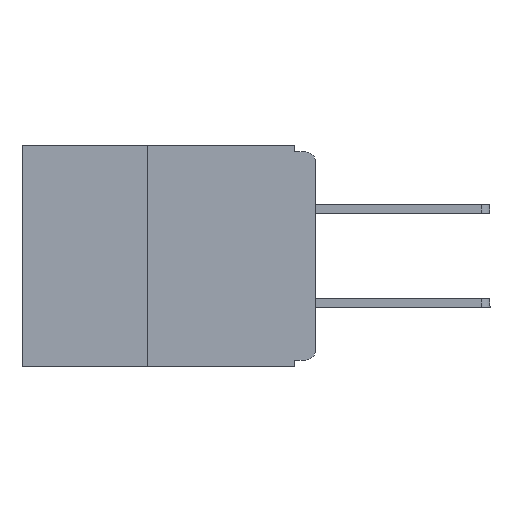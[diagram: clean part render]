
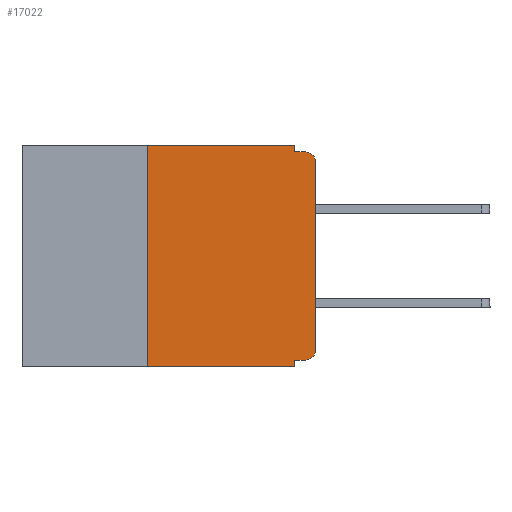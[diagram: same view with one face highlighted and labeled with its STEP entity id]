
A CAD part, left-side view. The second image highlights one B-rep face of the part: STEP entity #17022.
In plain terms, the highlighted planar face has unit normal (-1, 0, 0).
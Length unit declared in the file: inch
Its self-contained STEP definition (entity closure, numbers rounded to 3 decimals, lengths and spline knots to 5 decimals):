
#171 = DIRECTION ( 'NONE',  ( 0., 0., 1. ) ) ;
#229 = VERTEX_POINT ( 'NONE', #3097 ) ;
#685 = CARTESIAN_POINT ( 'NONE',  ( 0., 0., -0.305 ) ) ;
#747 = VERTEX_POINT ( 'NONE', #20195 ) ;
#1390 = ORIENTED_EDGE ( 'NONE', *, *, #5855, .T. ) ;
#1569 = PLANE ( 'NONE',  #25095 ) ;
#1769 = EDGE_CURVE ( 'NONE', #11417, #20608, #27484, .T. ) ;
#2028 = LINE ( 'NONE', #30187, #28240 ) ;
#2188 = EDGE_CURVE ( 'NONE', #27932, #9509, #2028, .T. ) ;
#2592 = LINE ( 'NONE', #24137, #16158 ) ;
#2807 = CIRCLE ( 'NONE', #29738, 0.015 ) ;
#3097 = CARTESIAN_POINT ( 'NONE',  ( 0., 0.031, -0.33 ) ) ;
#3810 = EDGE_CURVE ( 'NONE', #20608, #4296, #27402, .T. ) ;
#4108 = DIRECTION ( 'NONE',  ( 1., 0., 0. ) ) ;
#4151 = LINE ( 'NONE', #15385, #30288 ) ;
#4296 = VERTEX_POINT ( 'NONE', #9428 ) ;
#5158 = ORIENTED_EDGE ( 'NONE', *, *, #30270, .F. ) ;
#5855 = EDGE_CURVE ( 'NONE', #11417, #229, #32579, .T. ) ;
#6663 = CARTESIAN_POINT ( 'NONE',  ( 0., 0.25, -0.33 ) ) ;
#7225 = DIRECTION ( 'NONE',  ( -1., 0., 0. ) ) ;
#8771 = ORIENTED_EDGE ( 'NONE', *, *, #2188, .F. ) ;
#9335 = VERTEX_POINT ( 'NONE', #32453 ) ;
#9428 = CARTESIAN_POINT ( 'NONE',  ( 0., 0.031, 0. ) ) ;
#9509 = VERTEX_POINT ( 'NONE', #30810 ) ;
#9636 = ORIENTED_EDGE ( 'NONE', *, *, #11539, .T. ) ;
#10554 = FACE_OUTER_BOUND ( 'NONE', #23819, .T. ) ;
#10931 = DIRECTION ( 'NONE',  ( -1., 0., 0. ) ) ;
#11417 = VERTEX_POINT ( 'NONE', #6663 ) ;
#11539 = EDGE_CURVE ( 'NONE', #27932, #21836, #19241, .T. ) ;
#11646 = CARTESIAN_POINT ( 'NONE',  ( 0., 0.437, 0. ) ) ;
#12445 = CARTESIAN_POINT ( 'NONE',  ( 0., 0., -0.01 ) ) ;
#12714 = VECTOR ( 'NONE', #19038, 39.37008 ) ;
#12812 = CARTESIAN_POINT ( 'NONE',  ( 0., 0.031, -0.01 ) ) ;
#13519 = LINE ( 'NONE', #26538, #12714 ) ;
#13847 = VECTOR ( 'NONE', #20989, 39.37008 ) ;
#14106 = DIRECTION ( 'NONE',  ( 0., 1., 0. ) ) ;
#14584 = EDGE_CURVE ( 'NONE', #15882, #9335, #21091, .T. ) ;
#15385 = CARTESIAN_POINT ( 'NONE',  ( 0., 0., 0. ) ) ;
#15882 = VERTEX_POINT ( 'NONE', #12812 ) ;
#16158 = VECTOR ( 'NONE', #26626, 39.37008 ) ;
#16305 = ORIENTED_EDGE ( 'NONE', *, *, #14584, .F. ) ;
#17022 = ADVANCED_FACE ( 'NONE', ( #10554 ), #1569, .F. ) ;
#17591 = CARTESIAN_POINT ( 'NONE',  ( 0., 0.015, -0.32 ) ) ;
#19038 = DIRECTION ( 'NONE',  ( 0., 0., -1. ) ) ;
#19241 = CIRCLE ( 'NONE', #24144, 0.015 ) ;
#20195 = CARTESIAN_POINT ( 'NONE',  ( 0., 0., -0.025 ) ) ;
#20608 = VERTEX_POINT ( 'NONE', #26088 ) ;
#20829 = VECTOR ( 'NONE', #23068, 39.37008 ) ;
#20943 = CARTESIAN_POINT ( 'NONE',  ( 0., 0.437, 0. ) ) ;
#20989 = DIRECTION ( 'NONE',  ( 0., -1., 0. ) ) ;
#21091 = LINE ( 'NONE', #12445, #23723 ) ;
#21836 = VERTEX_POINT ( 'NONE', #685 ) ;
#21975 = DIRECTION ( 'NONE',  ( 0., 0., -1. ) ) ;
#22377 = ORIENTED_EDGE ( 'NONE', *, *, #3810, .F. ) ;
#22504 = CARTESIAN_POINT ( 'NONE',  ( 0., 0.25, -0.33 ) ) ;
#22537 = CARTESIAN_POINT ( 'NONE',  ( 0., 0.015, -0.305 ) ) ;
#22683 = ORIENTED_EDGE ( 'NONE', *, *, #30630, .T. ) ;
#23068 = DIRECTION ( 'NONE',  ( 0., 0., 1. ) ) ;
#23723 = VECTOR ( 'NONE', #30188, 39.37008 ) ;
#23819 = EDGE_LOOP ( 'NONE', ( #22683, #29535, #16305, #27939, #22377, #31810, #1390, #5158, #8771, #9636 ) ) ;
#23954 = EDGE_CURVE ( 'NONE', #4296, #15882, #13519, .T. ) ;
#24137 = CARTESIAN_POINT ( 'NONE',  ( 0., 0.031, -0.33 ) ) ;
#24144 = AXIS2_PLACEMENT_3D ( 'NONE', #22537, #7225, #25055 ) ;
#24508 = EDGE_CURVE ( 'NONE', #747, #9335, #2807, .T. ) ;
#25055 = DIRECTION ( 'NONE',  ( 0., 0., -1. ) ) ;
#25095 = AXIS2_PLACEMENT_3D ( 'NONE', #11646, #4108, #21975 ) ;
#26088 = CARTESIAN_POINT ( 'NONE',  ( 0., 0.25, 0. ) ) ;
#26189 = CARTESIAN_POINT ( 'NONE',  ( 0., 0.015, -0.025 ) ) ;
#26538 = CARTESIAN_POINT ( 'NONE',  ( 0., 0.031, 0. ) ) ;
#26626 = DIRECTION ( 'NONE',  ( 0., 0., -1. ) ) ;
#26894 = VECTOR ( 'NONE', #32262, 39.37008 ) ;
#27402 = LINE ( 'NONE', #20943, #13847 ) ;
#27484 = LINE ( 'NONE', #22504, #20829 ) ;
#27932 = VERTEX_POINT ( 'NONE', #17591 ) ;
#27939 = ORIENTED_EDGE ( 'NONE', *, *, #23954, .F. ) ;
#28240 = VECTOR ( 'NONE', #14106, 39.37008 ) ;
#28653 = DIRECTION ( 'NONE',  ( 0., 0., -1. ) ) ;
#29535 = ORIENTED_EDGE ( 'NONE', *, *, #24508, .T. ) ;
#29738 = AXIS2_PLACEMENT_3D ( 'NONE', #26189, #10931, #28653 ) ;
#30187 = CARTESIAN_POINT ( 'NONE',  ( 0., 0., -0.32 ) ) ;
#30188 = DIRECTION ( 'NONE',  ( 0., -1., 0. ) ) ;
#30270 = EDGE_CURVE ( 'NONE', #9509, #229, #2592, .T. ) ;
#30288 = VECTOR ( 'NONE', #171, 39.37008 ) ;
#30630 = EDGE_CURVE ( 'NONE', #21836, #747, #4151, .T. ) ;
#30810 = CARTESIAN_POINT ( 'NONE',  ( 0., 0.031, -0.32 ) ) ;
#31810 = ORIENTED_EDGE ( 'NONE', *, *, #1769, .F. ) ;
#32130 = CARTESIAN_POINT ( 'NONE',  ( 0., 0.437, -0.33 ) ) ;
#32262 = DIRECTION ( 'NONE',  ( 0., -1., 0. ) ) ;
#32453 = CARTESIAN_POINT ( 'NONE',  ( 0., 0.015, -0.01 ) ) ;
#32579 = LINE ( 'NONE', #32130, #26894 ) ;
